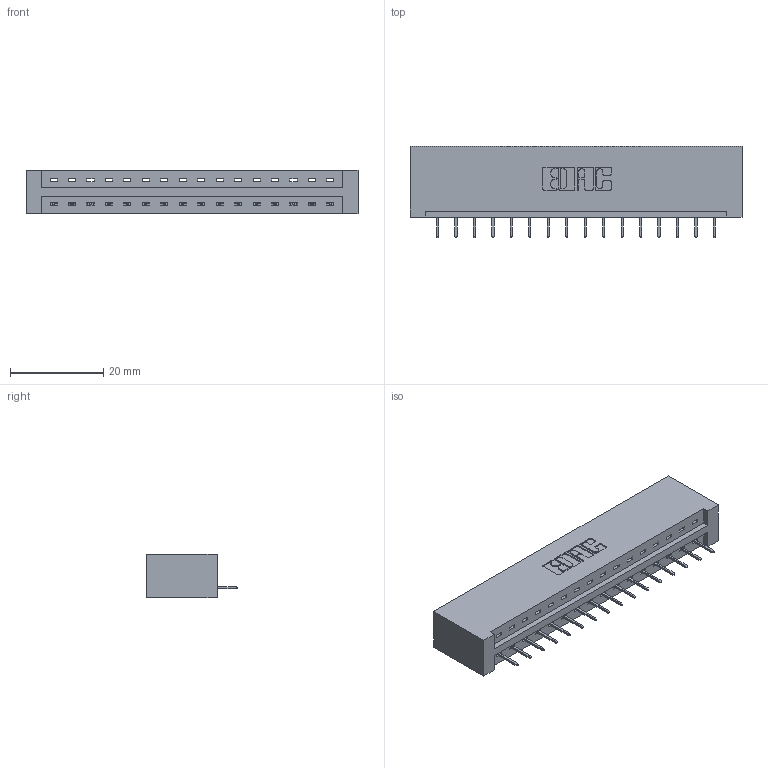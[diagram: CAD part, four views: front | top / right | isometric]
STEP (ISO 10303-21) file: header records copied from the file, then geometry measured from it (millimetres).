
FILE_DESCRIPTION (( 'STEP AP203' ), '1' );
FILE_NAME ('387-016-524-101.STEP', '2019-10-02T18:12:40', ( '' ), ( '' ), 'SwSTEP 2.0', 'SolidWorks 2016', '' );
FILE_SCHEMA (( 'CONFIG_CONTROL_DESIGN' ));
Length unit declared in the file: inch
Products named in the file (3): 345-292-001_345-293-124; 387-016-524-101; 337 Part_No Mounting Lugs
Assembly tree (17 placements, depth 2):
  387-016-524-101
    337 Part_No Mounting Lugs
    345-292-001_345-293-124  x16
Bounding box: 71.27 x 19.69 x 9.4 mm (x, y, z)
Volume: 7757.7 mm3; surface area: 7631.3 mm2
Topology: 17 solids, 17 shells, 1162 faces, 3359 edges, 2174 vertices
Faces by surface type: plane 898, cylinder 264
Entity records: 15053 total; most frequent: CARTESIAN_POINT 2626, ORIENTED_EDGE 2578, DIRECTION 2257, EDGE_CURVE 1289, LINE 1173, VECTOR 1173, VERTEX_POINT 854, AXIS2_PLACEMENT_3D 542
